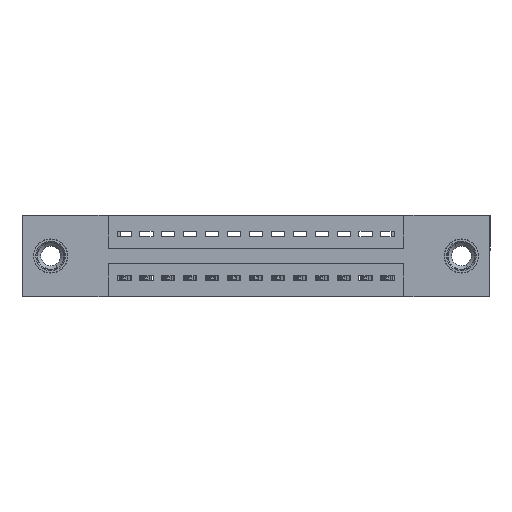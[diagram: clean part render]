
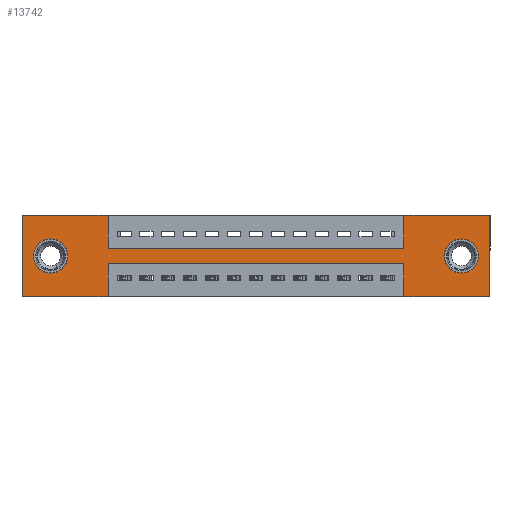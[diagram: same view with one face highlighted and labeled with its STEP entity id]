
A CAD part, front view. The second image highlights one B-rep face of the part: STEP entity #13742.
In plain terms, the highlighted planar face has unit normal (0, -1, 0).
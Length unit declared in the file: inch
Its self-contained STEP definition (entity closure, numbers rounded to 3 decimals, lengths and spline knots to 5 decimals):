
#34 = VERTEX_POINT ( 'NONE', #7796 ) ;
#663 = VECTOR ( 'NONE', #17309, 39.37008 ) ;
#715 = ORIENTED_EDGE ( 'NONE', *, *, #8997, .F. ) ;
#773 = DIRECTION ( 'NONE',  ( 1., 0., 0. ) ) ;
#942 = VERTEX_POINT ( 'NONE', #7269 ) ;
#1125 = VERTEX_POINT ( 'NONE', #3622 ) ;
#1167 = CARTESIAN_POINT ( 'NONE',  ( 2.005, 0., -0.185 ) ) ;
#1288 = EDGE_CURVE ( 'NONE', #17107, #9352, #13210, .T. ) ;
#1339 = DIRECTION ( 'NONE',  ( 0., 0., -1. ) ) ;
#1504 = EDGE_CURVE ( 'NONE', #1672, #942, #10520, .T. ) ;
#1600 = EDGE_CURVE ( 'NONE', #1125, #6173, #16298, .T. ) ;
#1672 = VERTEX_POINT ( 'NONE', #8255 ) ;
#1731 = EDGE_CURVE ( 'NONE', #2783, #11546, #12330, .T. ) ;
#1742 = ORIENTED_EDGE ( 'NONE', *, *, #1288, .F. ) ;
#1840 = VECTOR ( 'NONE', #8145, 39.37008 ) ;
#2026 = CARTESIAN_POINT ( 'NONE',  ( 1.7425, 0., 0. ) ) ;
#2382 = CARTESIAN_POINT ( 'NONE',  ( 2.135, 0., 0. ) ) ;
#2437 = DIRECTION ( 'NONE',  ( 0., 0., -1. ) ) ;
#2479 = EDGE_CURVE ( 'NONE', #13473, #15109, #16288, .T. ) ;
#2515 = VECTOR ( 'NONE', #5947, 39.37008 ) ;
#2588 = DIRECTION ( 'NONE',  ( 0., 1., 0. ) ) ;
#2617 = CARTESIAN_POINT ( 'NONE',  ( 1.7425, 0., -0.37 ) ) ;
#2783 = VERTEX_POINT ( 'NONE', #18054 ) ;
#2974 = CARTESIAN_POINT ( 'NONE',  ( 0., 0., -0.37 ) ) ;
#3211 = CARTESIAN_POINT ( 'NONE',  ( 0., 0., 0. ) ) ;
#3399 = LINE ( 'NONE', #5297, #1840 ) ;
#3499 = FACE_BOUND ( 'NONE', #11473, .T. ) ;
#3622 = CARTESIAN_POINT ( 'NONE',  ( 0.3925, 0., -0.37 ) ) ;
#3693 = EDGE_CURVE ( 'NONE', #16158, #4052, #15820, .T. ) ;
#3941 = CARTESIAN_POINT ( 'NONE',  ( 2.135, 0., -0.37 ) ) ;
#3988 = AXIS2_PLACEMENT_3D ( 'NONE', #4043, #15164, #13992 ) ;
#4043 = CARTESIAN_POINT ( 'NONE',  ( 0.13, 0., -0.185 ) ) ;
#4052 = VERTEX_POINT ( 'NONE', #15794 ) ;
#4389 = LINE ( 'NONE', #6072, #9055 ) ;
#4481 = ORIENTED_EDGE ( 'NONE', *, *, #1731, .F. ) ;
#4507 = EDGE_CURVE ( 'NONE', #6173, #34, #8507, .T. ) ;
#4556 = CARTESIAN_POINT ( 'NONE',  ( 0.3925, 0., 0. ) ) ;
#4579 = DIRECTION ( 'NONE',  ( -1., 0., 0. ) ) ;
#4640 = CARTESIAN_POINT ( 'NONE',  ( 0.3925, 0., -0.22 ) ) ;
#4868 = VERTEX_POINT ( 'NONE', #13790 ) ;
#5126 = CARTESIAN_POINT ( 'NONE',  ( 1.7425, 0., 0. ) ) ;
#5297 = CARTESIAN_POINT ( 'NONE',  ( 0.3925, 0., -0.37 ) ) ;
#5498 = VERTEX_POINT ( 'NONE', #14710 ) ;
#5729 = ORIENTED_EDGE ( 'NONE', *, *, #14553, .F. ) ;
#5800 = AXIS2_PLACEMENT_3D ( 'NONE', #17055, #15210, #1339 ) ;
#5947 = DIRECTION ( 'NONE',  ( -1., 0., 0. ) ) ;
#6072 = CARTESIAN_POINT ( 'NONE',  ( 0.3925, 0., -0.15 ) ) ;
#6170 = ORIENTED_EDGE ( 'NONE', *, *, #8200, .T. ) ;
#6173 = VERTEX_POINT ( 'NONE', #6879 ) ;
#6361 = CARTESIAN_POINT ( 'NONE',  ( 1.7425, 0., -0.37 ) ) ;
#6556 = DIRECTION ( 'NONE',  ( 0., 0., 1. ) ) ;
#6655 = VECTOR ( 'NONE', #9594, 39.37008 ) ;
#6879 = CARTESIAN_POINT ( 'NONE',  ( 0., 0., -0.37 ) ) ;
#6883 = EDGE_CURVE ( 'NONE', #12655, #4868, #11121, .T. ) ;
#6935 = CARTESIAN_POINT ( 'NONE',  ( 0.3925, 0., 0. ) ) ;
#6986 = AXIS2_PLACEMENT_3D ( 'NONE', #1167, #2588, #9747 ) ;
#7117 = ORIENTED_EDGE ( 'NONE', *, *, #11062, .T. ) ;
#7125 = CARTESIAN_POINT ( 'NONE',  ( 0.13, 0., -0.185 ) ) ;
#7269 = CARTESIAN_POINT ( 'NONE',  ( 2.005, 0., -0.107 ) ) ;
#7320 = ORIENTED_EDGE ( 'NONE', *, *, #4507, .F. ) ;
#7345 = ORIENTED_EDGE ( 'NONE', *, *, #1504, .T. ) ;
#7351 = CARTESIAN_POINT ( 'NONE',  ( 0., 0., 0. ) ) ;
#7380 = CIRCLE ( 'NONE', #7774, 0.078 ) ;
#7544 = LINE ( 'NONE', #8036, #6655 ) ;
#7774 = AXIS2_PLACEMENT_3D ( 'NONE', #15239, #10972, #2437 ) ;
#7796 = CARTESIAN_POINT ( 'NONE',  ( 0., 0., 0. ) ) ;
#7847 = EDGE_CURVE ( 'NONE', #4868, #2783, #4389, .T. ) ;
#7864 = DIRECTION ( 'NONE',  ( 0., 0., 1. ) ) ;
#8036 = CARTESIAN_POINT ( 'NONE',  ( 0., 0., 0. ) ) ;
#8145 = DIRECTION ( 'NONE',  ( 0., 0., -1. ) ) ;
#8200 = EDGE_CURVE ( 'NONE', #15109, #13473, #13733, .T. ) ;
#8233 = ORIENTED_EDGE ( 'NONE', *, *, #12482, .F. ) ;
#8255 = CARTESIAN_POINT ( 'NONE',  ( 2.005, 0., -0.263 ) ) ;
#8379 = EDGE_LOOP ( 'NONE', ( #7117, #7345 ) ) ;
#8413 = DIRECTION ( 'NONE',  ( 0., 0., -1. ) ) ;
#8452 = ORIENTED_EDGE ( 'NONE', *, *, #1600, .F. ) ;
#8507 = LINE ( 'NONE', #3211, #12516 ) ;
#8585 = LINE ( 'NONE', #10770, #17256 ) ;
#8997 = EDGE_CURVE ( 'NONE', #9352, #16158, #8585, .T. ) ;
#9055 = VECTOR ( 'NONE', #773, 39.37008 ) ;
#9114 = LINE ( 'NONE', #4640, #17785 ) ;
#9140 = VECTOR ( 'NONE', #12811, 39.37008 ) ;
#9352 = VERTEX_POINT ( 'NONE', #3941 ) ;
#9425 = VECTOR ( 'NONE', #8413, 39.37008 ) ;
#9594 = DIRECTION ( 'NONE',  ( 1., 0., 0. ) ) ;
#9747 = DIRECTION ( 'NONE',  ( 0., 0., -1. ) ) ;
#10413 = ORIENTED_EDGE ( 'NONE', *, *, #3693, .F. ) ;
#10481 = EDGE_CURVE ( 'NONE', #5498, #1125, #3399, .T. ) ;
#10520 = CIRCLE ( 'NONE', #6986, 0.078 ) ;
#10634 = CARTESIAN_POINT ( 'NONE',  ( 0.13, 0., -0.263 ) ) ;
#10770 = CARTESIAN_POINT ( 'NONE',  ( 0., 0., -0.37 ) ) ;
#10896 = VECTOR ( 'NONE', #12579, 39.37008 ) ;
#10900 = DIRECTION ( 'NONE',  ( -1., 0., 0. ) ) ;
#10910 = ORIENTED_EDGE ( 'NONE', *, *, #6883, .F. ) ;
#10972 = DIRECTION ( 'NONE',  ( 0., 1., 0. ) ) ;
#11062 = EDGE_CURVE ( 'NONE', #942, #1672, #7380, .T. ) ;
#11088 = FACE_BOUND ( 'NONE', #8379, .T. ) ;
#11121 = LINE ( 'NONE', #6935, #10896 ) ;
#11473 = EDGE_LOOP ( 'NONE', ( #6170, #17577 ) ) ;
#11546 = VERTEX_POINT ( 'NONE', #2026 ) ;
#12247 = EDGE_CURVE ( 'NONE', #34, #12655, #18284, .T. ) ;
#12330 = LINE ( 'NONE', #5126, #15655 ) ;
#12482 = EDGE_CURVE ( 'NONE', #4052, #5498, #9114, .T. ) ;
#12516 = VECTOR ( 'NONE', #7864, 39.37008 ) ;
#12579 = DIRECTION ( 'NONE',  ( 0., 0., -1. ) ) ;
#12655 = VERTEX_POINT ( 'NONE', #4556 ) ;
#12811 = DIRECTION ( 'NONE',  ( 0., 0., 1. ) ) ;
#13210 = LINE ( 'NONE', #2382, #9425 ) ;
#13284 = PLANE ( 'NONE',  #5800 ) ;
#13473 = VERTEX_POINT ( 'NONE', #10634 ) ;
#13733 = CIRCLE ( 'NONE', #17293, 0.078 ) ;
#13742 = ADVANCED_FACE ( 'NONE', ( #11088, #3499, #15962 ), #13284, .T. ) ;
#13790 = CARTESIAN_POINT ( 'NONE',  ( 0.3925, 0., -0.15 ) ) ;
#13992 = DIRECTION ( 'NONE',  ( 0., 0., 1. ) ) ;
#14553 = EDGE_CURVE ( 'NONE', #11546, #17107, #7544, .T. ) ;
#14710 = CARTESIAN_POINT ( 'NONE',  ( 0.3925, 0., -0.22 ) ) ;
#15109 = VERTEX_POINT ( 'NONE', #16783 ) ;
#15164 = DIRECTION ( 'NONE',  ( 0., 1., 0. ) ) ;
#15210 = DIRECTION ( 'NONE',  ( 0., -1., 0. ) ) ;
#15239 = CARTESIAN_POINT ( 'NONE',  ( 2.005, 0., -0.185 ) ) ;
#15623 = DIRECTION ( 'NONE',  ( 0., 1., 0. ) ) ;
#15643 = CARTESIAN_POINT ( 'NONE',  ( 2.135, 0., 0. ) ) ;
#15655 = VECTOR ( 'NONE', #6556, 39.37008 ) ;
#15794 = CARTESIAN_POINT ( 'NONE',  ( 1.7425, 0., -0.22 ) ) ;
#15820 = LINE ( 'NONE', #2617, #9140 ) ;
#15962 = FACE_OUTER_BOUND ( 'NONE', #16975, .T. ) ;
#16158 = VERTEX_POINT ( 'NONE', #6361 ) ;
#16288 = CIRCLE ( 'NONE', #3988, 0.078 ) ;
#16298 = LINE ( 'NONE', #2974, #2515 ) ;
#16508 = ORIENTED_EDGE ( 'NONE', *, *, #10481, .F. ) ;
#16783 = CARTESIAN_POINT ( 'NONE',  ( 0.13, 0., -0.107 ) ) ;
#16896 = ORIENTED_EDGE ( 'NONE', *, *, #7847, .F. ) ;
#16975 = EDGE_LOOP ( 'NONE', ( #16508, #8233, #10413, #715, #1742, #5729, #4481, #16896, #10910, #18205, #7320, #8452 ) ) ;
#17055 = CARTESIAN_POINT ( 'NONE',  ( 0., 0., -0.37 ) ) ;
#17073 = DIRECTION ( 'NONE',  ( 0., 0., 1. ) ) ;
#17107 = VERTEX_POINT ( 'NONE', #15643 ) ;
#17256 = VECTOR ( 'NONE', #10900, 39.37008 ) ;
#17293 = AXIS2_PLACEMENT_3D ( 'NONE', #7125, #15623, #17073 ) ;
#17309 = DIRECTION ( 'NONE',  ( 1., 0., 0. ) ) ;
#17577 = ORIENTED_EDGE ( 'NONE', *, *, #2479, .T. ) ;
#17785 = VECTOR ( 'NONE', #4579, 39.37008 ) ;
#18054 = CARTESIAN_POINT ( 'NONE',  ( 1.7425, 0., -0.15 ) ) ;
#18205 = ORIENTED_EDGE ( 'NONE', *, *, #12247, .F. ) ;
#18284 = LINE ( 'NONE', #7351, #663 ) ;
